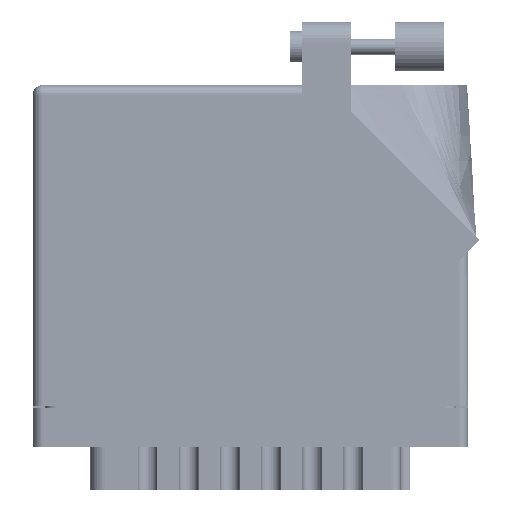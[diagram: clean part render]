
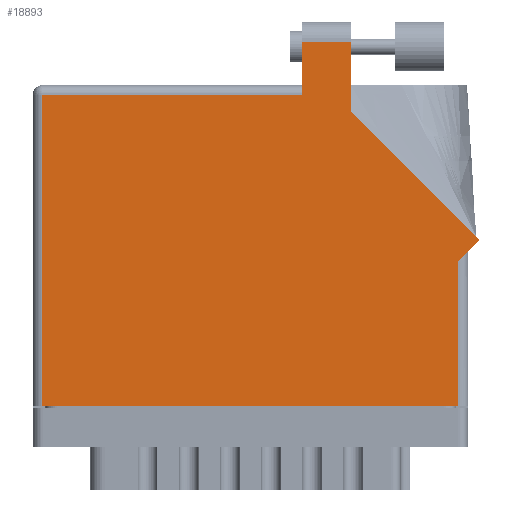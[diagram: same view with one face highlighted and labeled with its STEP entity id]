
A CAD part, front view. The second image highlights one B-rep face of the part: STEP entity #18893.
In plain terms, the highlighted face is planar.
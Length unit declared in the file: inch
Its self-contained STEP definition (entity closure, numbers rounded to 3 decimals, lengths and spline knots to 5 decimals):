
#2276 = CARTESIAN_POINT ( 'NONE',  ( 1.705, 2.305, 0. ) ) ;
#2378 = VERTEX_POINT ( 'NONE', #48475 ) ;
#3184 = EDGE_CURVE ( 'NONE', #51321, #57984, #84465, .T. ) ;
#6287 = CARTESIAN_POINT ( 'NONE',  ( 2.693, 0.918, 0. ) ) ;
#9656 = DIRECTION ( 'NONE',  ( -1., 0., 0. ) ) ;
#10140 = LINE ( 'NONE', #30362, #71043 ) ;
#13639 = ORIENTED_EDGE ( 'NONE', *, *, #29588, .T. ) ;
#13781 = CARTESIAN_POINT ( 'NONE',  ( 2.693, 0.98, 0. ) ) ;
#14133 = EDGE_CURVE ( 'NONE', #2378, #39614, #85420, .T. ) ;
#14642 = VECTOR ( 'NONE', #91480, 39.37008 ) ;
#18893 = ADVANCED_FACE ( 'NONE', ( #84129 ), #19668, .F. ) ;
#19326 = ORIENTED_EDGE ( 'NONE', *, *, #79623, .T. ) ;
#19668 = PLANE ( 'NONE',  #63211 ) ;
#20794 = EDGE_CURVE ( 'NONE', #70496, #49162, #10140, .T. ) ;
#23289 = ORIENTED_EDGE ( 'NONE', *, *, #62887, .T. ) ;
#24156 = ORIENTED_EDGE ( 'NONE', *, *, #3184, .T. ) ;
#26112 = LINE ( 'NONE', #2276, #59251 ) ;
#29588 = EDGE_CURVE ( 'NONE', #34431, #2378, #84717, .T. ) ;
#30362 = CARTESIAN_POINT ( 'NONE',  ( 1.705, 2.03, 0. ) ) ;
#34431 = VERTEX_POINT ( 'NONE', #88903 ) ;
#34546 = VECTOR ( 'NONE', #56735, 39.37008 ) ;
#37850 = CARTESIAN_POINT ( 'NONE',  ( 2.012, 1.86442, 0. ) ) ;
#38829 = DIRECTION ( 'NONE',  ( 0., -1., 0. ) ) ;
#39453 = LINE ( 'NONE', #46052, #70549 ) ;
#39614 = VERTEX_POINT ( 'NONE', #64944 ) ;
#39853 = ORIENTED_EDGE ( 'NONE', *, *, #52936, .T. ) ;
#41156 = LINE ( 'NONE', #69835, #14642 ) ;
#41616 = CARTESIAN_POINT ( 'NONE',  ( 1.705, 2.305, 0. ) ) ;
#41914 = DIRECTION ( 'NONE',  ( 0., -1., 0. ) ) ;
#42440 = VECTOR ( 'NONE', #58465, 39.37008 ) ;
#43077 = CARTESIAN_POINT ( 'NONE',  ( 2.012, 1.86442, 0. ) ) ;
#44214 = ORIENTED_EDGE ( 'NONE', *, *, #76717, .T. ) ;
#45078 = VERTEX_POINT ( 'NONE', #71124 ) ;
#46052 = CARTESIAN_POINT ( 'NONE',  ( 0., 1.968, 0. ) ) ;
#48373 = CARTESIAN_POINT ( 'NONE',  ( 0., 2.03, 0. ) ) ;
#48475 = CARTESIAN_POINT ( 'NONE',  ( 0.062, 0., 0. ) ) ;
#49162 = VERTEX_POINT ( 'NONE', #77246 ) ;
#49628 = CARTESIAN_POINT ( 'NONE',  ( 2.012, 2.305, 0. ) ) ;
#49630 = VECTOR ( 'NONE', #41914, 39.37008 ) ;
#51062 = CARTESIAN_POINT ( 'NONE',  ( 0., 0., 0. ) ) ;
#51321 = VERTEX_POINT ( 'NONE', #37850 ) ;
#51544 = DIRECTION ( 'NONE',  ( 0., 0., -1. ) ) ;
#52936 = EDGE_CURVE ( 'NONE', #92797, #45078, #41156, .T. ) ;
#53798 = EDGE_LOOP ( 'NONE', ( #24156, #23289, #67004, #44214, #13639, #70134, #58704, #39853, #19326 ) ) ;
#56045 = CARTESIAN_POINT ( 'NONE',  ( 0.062, 0., 0. ) ) ;
#56154 = LINE ( 'NONE', #13781, #42440 ) ;
#56735 = DIRECTION ( 'NONE',  ( 0., 1., 0. ) ) ;
#56754 = DIRECTION ( 'NONE',  ( 1., 0., 0. ) ) ;
#57984 = VERTEX_POINT ( 'NONE', #49628 ) ;
#58465 = DIRECTION ( 'NONE',  ( 0., 1., 0. ) ) ;
#58704 = ORIENTED_EDGE ( 'NONE', *, *, #59813, .T. ) ;
#59251 = VECTOR ( 'NONE', #62355, 39.37008 ) ;
#59813 = EDGE_CURVE ( 'NONE', #39614, #92797, #56154, .T. ) ;
#62355 = DIRECTION ( 'NONE',  ( -1., 0., 0. ) ) ;
#62887 = EDGE_CURVE ( 'NONE', #57984, #70496, #26112, .T. ) ;
#63211 = AXIS2_PLACEMENT_3D ( 'NONE', #48373, #51544, #9656 ) ;
#64944 = CARTESIAN_POINT ( 'NONE',  ( 2.693, 0., 0. ) ) ;
#65796 = DIRECTION ( 'NONE',  ( -0.707, 0.707, 0. ) ) ;
#67004 = ORIENTED_EDGE ( 'NONE', *, *, #20794, .T. ) ;
#68468 = LINE ( 'NONE', #90115, #87544 ) ;
#69835 = CARTESIAN_POINT ( 'NONE',  ( 2.755, 0.98, 0. ) ) ;
#70134 = ORIENTED_EDGE ( 'NONE', *, *, #14133, .T. ) ;
#70496 = VERTEX_POINT ( 'NONE', #41616 ) ;
#70549 = VECTOR ( 'NONE', #81792, 39.37008 ) ;
#70787 = VECTOR ( 'NONE', #56754, 39.37008 ) ;
#71043 = VECTOR ( 'NONE', #38829, 39.37008 ) ;
#71124 = CARTESIAN_POINT ( 'NONE',  ( 2.82571, 1.05071, 0. ) ) ;
#76717 = EDGE_CURVE ( 'NONE', #49162, #34431, #39453, .T. ) ;
#77246 = CARTESIAN_POINT ( 'NONE',  ( 1.705, 1.968, 0. ) ) ;
#79623 = EDGE_CURVE ( 'NONE', #45078, #51321, #68468, .T. ) ;
#81792 = DIRECTION ( 'NONE',  ( -1., 0., 0. ) ) ;
#84129 = FACE_OUTER_BOUND ( 'NONE', #53798, .T. ) ;
#84465 = LINE ( 'NONE', #43077, #34546 ) ;
#84717 = LINE ( 'NONE', #56045, #49630 ) ;
#85420 = LINE ( 'NONE', #51062, #70787 ) ;
#87544 = VECTOR ( 'NONE', #65796, 39.37008 ) ;
#88903 = CARTESIAN_POINT ( 'NONE',  ( 0.062, 1.968, 0. ) ) ;
#90115 = CARTESIAN_POINT ( 'NONE',  ( 2.82571, 1.05071, 0. ) ) ;
#91480 = DIRECTION ( 'NONE',  ( 0.707, 0.707, 0. ) ) ;
#92797 = VERTEX_POINT ( 'NONE', #6287 ) ;
